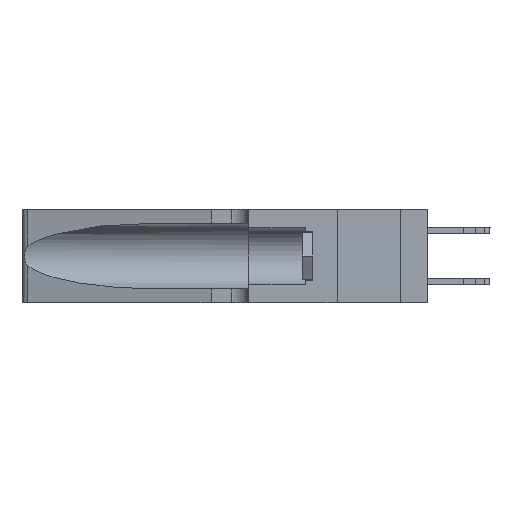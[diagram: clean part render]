
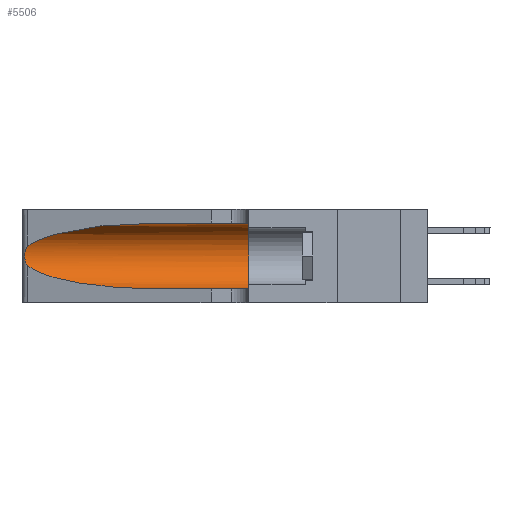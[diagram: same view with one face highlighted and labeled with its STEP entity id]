
A CAD part, left-side view. The second image highlights one B-rep face of the part: STEP entity #5506.
In plain terms, the highlighted cylindrical face has radius 3.308 mm (diameter 6.617 mm), a partial arc.
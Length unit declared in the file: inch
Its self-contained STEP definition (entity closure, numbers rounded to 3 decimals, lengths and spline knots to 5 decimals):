
#293 = FACE_OUTER_BOUND ( 'NONE', #21567, .T. ) ;
#1308 = EDGE_CURVE ( 'NONE', #15894, #14958, #6584, .T. ) ;
#1390 =( BOUNDED_CURVE ( )  B_SPLINE_CURVE ( 3, ( #4659, #6356, #2784, #9876 ),
 .UNSPECIFIED., .F., .T. ) 
 B_SPLINE_CURVE_WITH_KNOTS ( ( 4, 4 ),
 ( 3.44316, 4.71239 ),
 .UNSPECIFIED. ) 
 CURVE ( )  GEOMETRIC_REPRESENTATION_ITEM ( )  RATIONAL_B_SPLINE_CURVE ( ( 1., 0.87, 0.87, 1. ) ) 
 REPRESENTATION_ITEM ( '' )  );
#1484 = CARTESIAN_POINT ( 'NONE',  ( 0.25639, 1.23184, 0.21858 ) ) ;
#1849 = LINE ( 'NONE', #5639, #14809 ) ;
#1965 = CARTESIAN_POINT ( 'NONE',  ( 0.1305, 0.72297, 0.05475 ) ) ;
#2101 = EDGE_CURVE ( 'NONE', #15796, #13141, #1849, .T. ) ;
#2523 = CARTESIAN_POINT ( 'NONE',  ( 0.18966, 0.96281, 0.31525 ) ) ;
#2648 = ORIENTED_EDGE ( 'NONE', *, *, #1308, .T. ) ;
#2784 = CARTESIAN_POINT ( 'NONE',  ( 0.18966, 0.96281, 0.05475 ) ) ;
#3114 = CARTESIAN_POINT ( 'NONE',  ( 0.26075, 1.23896, 0.19203 ) ) ;
#3267 = CARTESIAN_POINT ( 'NONE',  ( 0.26018, 1.23835, 0.19895 ) ) ;
#3376 = CARTESIAN_POINT ( 'NONE',  ( 0.25487, 1.22718, 0.14631 ) ) ;
#3752 = DIRECTION ( 'NONE',  ( 0., -1., 0. ) ) ;
#4353 = CARTESIAN_POINT ( 'NONE',  ( 0.1305, 0.35, 0.31525 ) ) ;
#4588 = ORIENTED_EDGE ( 'NONE', *, *, #15422, .F. ) ;
#4659 = CARTESIAN_POINT ( 'NONE',  ( 0.25487, 1.22718, 0.14631 ) ) ;
#5061 = CARTESIAN_POINT ( 'NONE',  ( 0.26075, 1.23896, 0.178 ) ) ;
#5083 = LINE ( 'NONE', #19584, #18602 ) ;
#5506 = ADVANCED_FACE ( 'NONE', ( #293 ), #21320, .F. ) ;
#5639 = CARTESIAN_POINT ( 'NONE',  ( 0.1305, 1.61858, 0.05475 ) ) ;
#6013 = CARTESIAN_POINT ( 'NONE',  ( 0.1305, 0.72297, 0.31525 ) ) ;
#6163 = CARTESIAN_POINT ( 'NONE',  ( 0.25487, 1.22718, 0.22369 ) ) ;
#6356 = CARTESIAN_POINT ( 'NONE',  ( 0.2373, 1.15595, 0.08982 ) ) ;
#6584 =( BOUNDED_CURVE ( )  B_SPLINE_CURVE ( 3, ( #6013, #2523, #21887, #6163 ),
 .UNSPECIFIED., .F., .F. ) 
 B_SPLINE_CURVE_WITH_KNOTS ( ( 4, 4 ),
 ( 1.5708, 2.84003 ),
 .UNSPECIFIED. ) 
 CURVE ( )  GEOMETRIC_REPRESENTATION_ITEM ( )  RATIONAL_B_SPLINE_CURVE ( ( 1., 0.87, 0.87, 1. ) ) 
 REPRESENTATION_ITEM ( '' )  );
#6745 = CARTESIAN_POINT ( 'NONE',  ( 0.25555, 1.22994, 0.2215 ) ) ;
#6825 = CARTESIAN_POINT ( 'NONE',  ( 0.26017, 1.23833, 0.17102 ) ) ;
#6974 = DIRECTION ( 'NONE',  ( 0., 0., -1. ) ) ;
#8566 = CARTESIAN_POINT ( 'NONE',  ( 0.25639, 1.23186, 0.15144 ) ) ;
#9160 = DIRECTION ( 'NONE',  ( 0., -1., 0. ) ) ;
#9184 = ORIENTED_EDGE ( 'NONE', *, *, #2101, .T. ) ;
#9876 = CARTESIAN_POINT ( 'NONE',  ( 0.1305, 0.72297, 0.05475 ) ) ;
#9955 = CIRCLE ( 'NONE', #11726, 0.13025 ) ;
#11379 = EDGE_CURVE ( 'NONE', #11527, #15796, #1390, .T. ) ;
#11527 = VERTEX_POINT ( 'NONE', #3376 ) ;
#11726 = AXIS2_PLACEMENT_3D ( 'NONE', #13129, #22204, #14909 ) ;
#13129 = CARTESIAN_POINT ( 'NONE',  ( 0.1305, 0.35, 0.185 ) ) ;
#13141 = VERTEX_POINT ( 'NONE', #15126 ) ;
#13829 = CARTESIAN_POINT ( 'NONE',  ( 0.25854, 1.2359, 0.20912 ) ) ;
#14809 = VECTOR ( 'NONE', #9160, 39.37008 ) ;
#14909 = DIRECTION ( 'NONE',  ( 0., 0., 1. ) ) ;
#14958 = VERTEX_POINT ( 'NONE', #16677 ) ;
#15114 = VERTEX_POINT ( 'NONE', #4353 ) ;
#15126 = CARTESIAN_POINT ( 'NONE',  ( 0.1305, 0.35, 0.05475 ) ) ;
#15422 = EDGE_CURVE ( 'NONE', #15894, #15114, #5083, .T. ) ;
#15449 = CARTESIAN_POINT ( 'NONE',  ( 0.25856, 1.23593, 0.16098 ) ) ;
#15459 = AXIS2_PLACEMENT_3D ( 'NONE', #17554, #22652, #6974 ) ;
#15796 = VERTEX_POINT ( 'NONE', #1965 ) ;
#15894 = VERTEX_POINT ( 'NONE', #15914 ) ;
#15914 = CARTESIAN_POINT ( 'NONE',  ( 0.1305, 0.72297, 0.31525 ) ) ;
#16677 = CARTESIAN_POINT ( 'NONE',  ( 0.25487, 1.22718, 0.22369 ) ) ;
#16686 = ORIENTED_EDGE ( 'NONE', *, *, #11379, .T. ) ;
#16745 = ORIENTED_EDGE ( 'NONE', *, *, #19787, .T. ) ;
#17078 = CARTESIAN_POINT ( 'NONE',  ( 0.25787, 1.23484, 0.2124 ) ) ;
#17387 = CARTESIAN_POINT ( 'NONE',  ( 0.25789, 1.23486, 0.15765 ) ) ;
#17554 = CARTESIAN_POINT ( 'NONE',  ( 0.1305, 1.61858, 0.185 ) ) ;
#18602 = VECTOR ( 'NONE', #3752, 39.37008 ) ;
#18886 = CARTESIAN_POINT ( 'NONE',  ( 0.25487, 1.22718, 0.14631 ) ) ;
#19584 = CARTESIAN_POINT ( 'NONE',  ( 0.1305, 1.61858, 0.31525 ) ) ;
#19787 = EDGE_CURVE ( 'NONE', #14958, #11527, #21885, .T. ) ;
#21320 = CYLINDRICAL_SURFACE ( 'NONE', #15459, 0.13025 ) ;
#21497 = EDGE_CURVE ( 'NONE', #15114, #13141, #9955, .T. ) ;
#21567 = EDGE_LOOP ( 'NONE', ( #2648, #16745, #16686, #9184, #22648, #4588 ) ) ;
#21885 = B_SPLINE_CURVE_WITH_KNOTS ( 'NONE', 3,
 ( #22642, #6745, #1484, #17078, #13829, #3267, #3114, #5061, #6825, #15449, #17387, #8566, #22359, #18886 ),
 .UNSPECIFIED., .F., .F.,
 ( 4, 2, 2, 2, 2, 2, 4 ),
 ( 0., 0.00027, 0.00053, 0.00107, 0.0016, 0.00187, 0.00214 ),
 .UNSPECIFIED. ) ;
#21887 = CARTESIAN_POINT ( 'NONE',  ( 0.2373, 1.15595, 0.28018 ) ) ;
#22204 = DIRECTION ( 'NONE',  ( 0., 1., 0. ) ) ;
#22359 = CARTESIAN_POINT ( 'NONE',  ( 0.25555, 1.22993, 0.14849 ) ) ;
#22642 = CARTESIAN_POINT ( 'NONE',  ( 0.25487, 1.22718, 0.22369 ) ) ;
#22648 = ORIENTED_EDGE ( 'NONE', *, *, #21497, .F. ) ;
#22652 = DIRECTION ( 'NONE',  ( 0., -1., 0. ) ) ;
